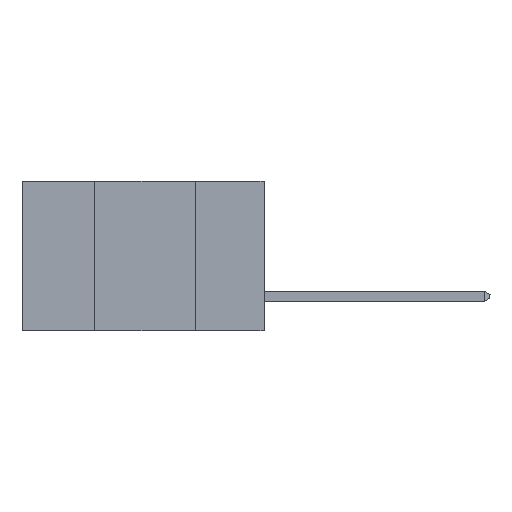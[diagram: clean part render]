
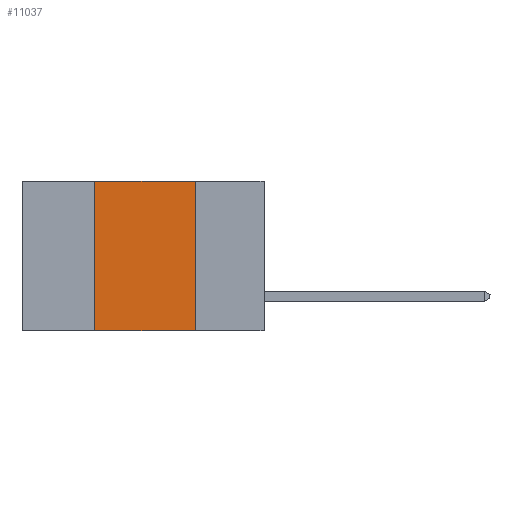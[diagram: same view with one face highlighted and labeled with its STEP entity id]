
A CAD part, left-side view. The second image highlights one B-rep face of the part: STEP entity #11037.
In plain terms, the highlighted planar face has unit normal (-1, 0, 0).
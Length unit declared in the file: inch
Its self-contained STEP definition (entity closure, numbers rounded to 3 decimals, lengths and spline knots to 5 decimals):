
#805 = FACE_OUTER_BOUND ( 'NONE', #13474, .T. ) ;
#915 = VECTOR ( 'NONE', #3411, 39.37008 ) ;
#1167 = LINE ( 'NONE', #9956, #8949 ) ;
#1542 = DIRECTION ( 'NONE',  ( 0., -1., 0. ) ) ;
#1877 = EDGE_CURVE ( 'NONE', #13215, #14267, #1167, .T. ) ;
#2086 = DIRECTION ( 'NONE',  ( 0., 0., 1. ) ) ;
#2251 = CARTESIAN_POINT ( 'NONE',  ( 0., 0.17, -0.37 ) ) ;
#2907 = EDGE_CURVE ( 'NONE', #7879, #6658, #8259, .T. ) ;
#3411 = DIRECTION ( 'NONE',  ( 0., 0., -1. ) ) ;
#3888 = CARTESIAN_POINT ( 'NONE',  ( 0., 0.6, 0. ) ) ;
#4305 = EDGE_CURVE ( 'NONE', #6658, #14267, #12151, .T. ) ;
#4321 = CARTESIAN_POINT ( 'NONE',  ( 0., 0.42, 0. ) ) ;
#5221 = VECTOR ( 'NONE', #2086, 39.37008 ) ;
#5226 = DIRECTION ( 'NONE',  ( 1., 0., 0. ) ) ;
#5463 = CARTESIAN_POINT ( 'NONE',  ( 0., 0.42, -0.37 ) ) ;
#5650 = AXIS2_PLACEMENT_3D ( 'NONE', #11779, #5226, #9670 ) ;
#6169 = PLANE ( 'NONE',  #5650 ) ;
#6658 = VERTEX_POINT ( 'NONE', #7224 ) ;
#7224 = CARTESIAN_POINT ( 'NONE',  ( 0., 0.17, 0. ) ) ;
#7242 = ORIENTED_EDGE ( 'NONE', *, *, #2907, .F. ) ;
#7275 = CARTESIAN_POINT ( 'NONE',  ( 0., 0.17, -0.37 ) ) ;
#7416 = CARTESIAN_POINT ( 'NONE',  ( 0., 0.42, -0.37 ) ) ;
#7879 = VERTEX_POINT ( 'NONE', #4321 ) ;
#8259 = LINE ( 'NONE', #3888, #14264 ) ;
#8876 = DIRECTION ( 'NONE',  ( 0., -1., 0. ) ) ;
#8949 = VECTOR ( 'NONE', #8876, 39.37008 ) ;
#9405 = ORIENTED_EDGE ( 'NONE', *, *, #11177, .F. ) ;
#9670 = DIRECTION ( 'NONE',  ( 0., 0., -1. ) ) ;
#9956 = CARTESIAN_POINT ( 'NONE',  ( 0., 0.6, -0.37 ) ) ;
#11037 = ADVANCED_FACE ( 'NONE', ( #805 ), #6169, .F. ) ;
#11101 = ORIENTED_EDGE ( 'NONE', *, *, #1877, .T. ) ;
#11177 = EDGE_CURVE ( 'NONE', #13215, #7879, #14122, .T. ) ;
#11779 = CARTESIAN_POINT ( 'NONE',  ( 0., 0.6, 0. ) ) ;
#11853 = ORIENTED_EDGE ( 'NONE', *, *, #4305, .F. ) ;
#12151 = LINE ( 'NONE', #2251, #915 ) ;
#13215 = VERTEX_POINT ( 'NONE', #7416 ) ;
#13474 = EDGE_LOOP ( 'NONE', ( #11853, #7242, #9405, #11101 ) ) ;
#14122 = LINE ( 'NONE', #5463, #5221 ) ;
#14264 = VECTOR ( 'NONE', #1542, 39.37008 ) ;
#14267 = VERTEX_POINT ( 'NONE', #7275 ) ;
